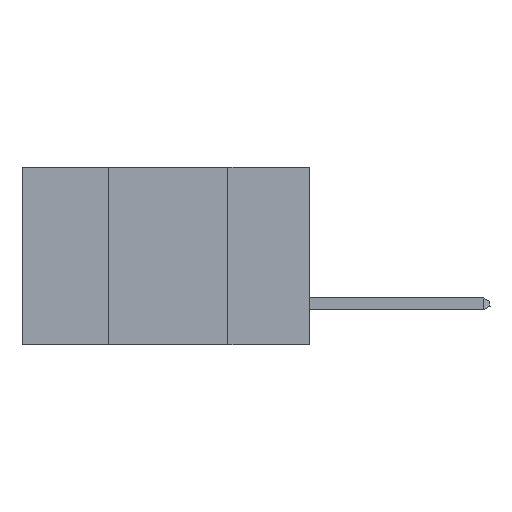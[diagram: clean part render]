
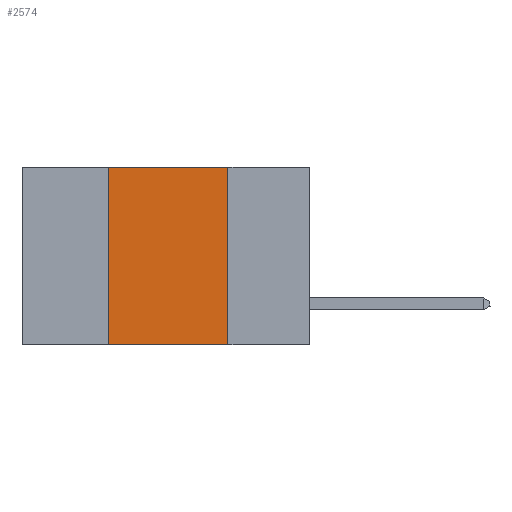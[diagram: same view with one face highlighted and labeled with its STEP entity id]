
A CAD part, left-side view. The second image highlights one B-rep face of the part: STEP entity #2574.
In plain terms, the highlighted planar face has unit normal (-1, 0, 0).
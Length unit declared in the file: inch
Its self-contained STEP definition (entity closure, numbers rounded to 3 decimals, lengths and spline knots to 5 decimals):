
#32 = DIRECTION ( 'NONE',  ( 1., 0., 0. ) ) ;
#176 = CARTESIAN_POINT ( 'NONE',  ( 0., 0.6, 0. ) ) ;
#672 = LINE ( 'NONE', #862, #6519 ) ;
#850 = EDGE_CURVE ( 'NONE', #3463, #15546, #10516, .T. ) ;
#862 = CARTESIAN_POINT ( 'NONE',  ( 0., 0.42, 0. ) ) ;
#1075 = VECTOR ( 'NONE', #4955, 39.37008 ) ;
#1189 = DIRECTION ( 'NONE',  ( 0., -1., 0. ) ) ;
#1267 = DIRECTION ( 'NONE',  ( 0., 0., -1. ) ) ;
#1417 = EDGE_CURVE ( 'NONE', #7506, #15546, #10154, .T. ) ;
#2117 = VECTOR ( 'NONE', #1189, 39.37008 ) ;
#2352 = CARTESIAN_POINT ( 'NONE',  ( 0., 0.17, 0. ) ) ;
#2400 = DIRECTION ( 'NONE',  ( 0., 0., -1. ) ) ;
#2545 = DIRECTION ( 'NONE',  ( 0., 0., 1. ) ) ;
#2574 = ADVANCED_FACE ( 'NONE', ( #5377 ), #7452, .F. ) ;
#3044 = AXIS2_PLACEMENT_3D ( 'NONE', #176, #32, #1267 ) ;
#3422 = EDGE_CURVE ( 'NONE', #4254, #3463, #14239, .T. ) ;
#3463 = VERTEX_POINT ( 'NONE', #7313 ) ;
#3663 = CARTESIAN_POINT ( 'NONE',  ( 0., 0.6, -0.37 ) ) ;
#4254 = VERTEX_POINT ( 'NONE', #5513 ) ;
#4820 = CARTESIAN_POINT ( 'NONE',  ( 0., 0.17, -0.37 ) ) ;
#4955 = DIRECTION ( 'NONE',  ( 0., -1., 0. ) ) ;
#5377 = FACE_OUTER_BOUND ( 'NONE', #14311, .T. ) ;
#5513 = CARTESIAN_POINT ( 'NONE',  ( 0., 0.42, 0. ) ) ;
#5784 = VECTOR ( 'NONE', #2400, 39.37008 ) ;
#6329 = ORIENTED_EDGE ( 'NONE', *, *, #1417, .T. ) ;
#6409 = ORIENTED_EDGE ( 'NONE', *, *, #10085, .F. ) ;
#6519 = VECTOR ( 'NONE', #2545, 39.37008 ) ;
#7255 = CARTESIAN_POINT ( 'NONE',  ( 0., 0.6, 0. ) ) ;
#7313 = CARTESIAN_POINT ( 'NONE',  ( 0., 0.17, 0. ) ) ;
#7452 = PLANE ( 'NONE',  #3044 ) ;
#7506 = VERTEX_POINT ( 'NONE', #13778 ) ;
#10085 = EDGE_CURVE ( 'NONE', #7506, #4254, #672, .T. ) ;
#10154 = LINE ( 'NONE', #3663, #1075 ) ;
#10516 = LINE ( 'NONE', #2352, #5784 ) ;
#11625 = ORIENTED_EDGE ( 'NONE', *, *, #850, .F. ) ;
#13778 = CARTESIAN_POINT ( 'NONE',  ( 0., 0.42, -0.37 ) ) ;
#14239 = LINE ( 'NONE', #7255, #2117 ) ;
#14311 = EDGE_LOOP ( 'NONE', ( #11625, #14602, #6409, #6329 ) ) ;
#14602 = ORIENTED_EDGE ( 'NONE', *, *, #3422, .F. ) ;
#15546 = VERTEX_POINT ( 'NONE', #4820 ) ;
